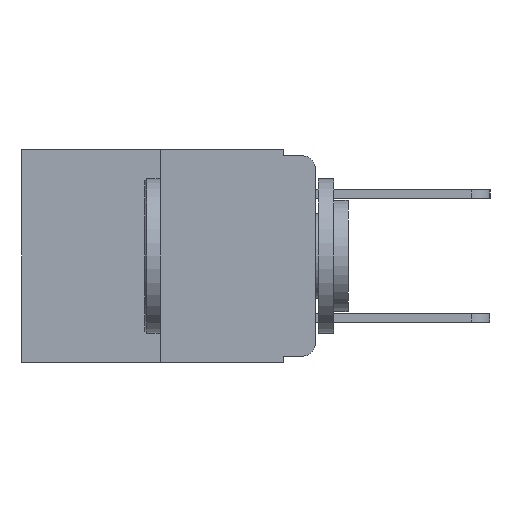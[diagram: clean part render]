
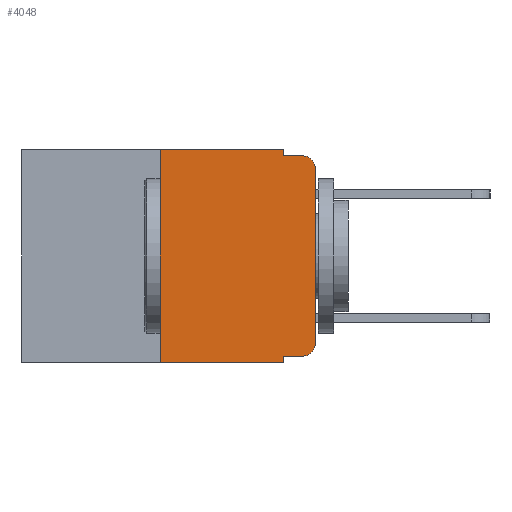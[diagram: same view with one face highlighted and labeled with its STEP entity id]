
A CAD part, left-side view. The second image highlights one B-rep face of the part: STEP entity #4048.
In plain terms, the highlighted planar face has unit normal (-1, 0, 0).
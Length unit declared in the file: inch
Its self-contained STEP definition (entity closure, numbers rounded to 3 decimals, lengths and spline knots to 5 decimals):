
#87 = DIRECTION ( 'NONE',  ( -1., 0., 0. ) ) ;
#447 = EDGE_CURVE ( 'NONE', #23786, #11235, #17488, .T. ) ;
#547 = ORIENTED_EDGE ( 'NONE', *, *, #9632, .F. ) ;
#900 = CARTESIAN_POINT ( 'NONE',  ( 0., 0.02, -0.01 ) ) ;
#1013 = EDGE_CURVE ( 'NONE', #1791, #23786, #21207, .T. ) ;
#1163 = CARTESIAN_POINT ( 'NONE',  ( 0., 0.473, 0. ) ) ;
#1171 = ORIENTED_EDGE ( 'NONE', *, *, #13634, .T. ) ;
#1400 = EDGE_CURVE ( 'NONE', #11235, #16687, #11119, .T. ) ;
#1454 = ORIENTED_EDGE ( 'NONE', *, *, #5997, .F. ) ;
#1662 = CARTESIAN_POINT ( 'NONE',  ( 0., 0.473, 0. ) ) ;
#1791 = VERTEX_POINT ( 'NONE', #5552 ) ;
#1856 = DIRECTION ( 'NONE',  ( 0., 0., -1. ) ) ;
#2005 = CARTESIAN_POINT ( 'NONE',  ( 0., 0.25, -0.343 ) ) ;
#2042 = DIRECTION ( 'NONE',  ( 0., 0., 1. ) ) ;
#2281 = AXIS2_PLACEMENT_3D ( 'NONE', #1163, #19923, #8902 ) ;
#2960 = CARTESIAN_POINT ( 'NONE',  ( 0., 0.051, -0.01 ) ) ;
#3100 = CARTESIAN_POINT ( 'NONE',  ( 0., 0., -0.313 ) ) ;
#3268 = ORIENTED_EDGE ( 'NONE', *, *, #447, .T. ) ;
#3965 = VERTEX_POINT ( 'NONE', #21559 ) ;
#4048 = ADVANCED_FACE ( 'NONE', ( #5320 ), #18096, .F. ) ;
#4071 = VECTOR ( 'NONE', #14919, 39.37008 ) ;
#4297 = CARTESIAN_POINT ( 'NONE',  ( 0., 0., -0.03 ) ) ;
#4522 = CARTESIAN_POINT ( 'NONE',  ( 0., 0., 0. ) ) ;
#4771 = EDGE_CURVE ( 'NONE', #18397, #10163, #5593, .T. ) ;
#5320 = FACE_OUTER_BOUND ( 'NONE', #21579, .T. ) ;
#5395 = CARTESIAN_POINT ( 'NONE',  ( 0., 0.02, -0.03 ) ) ;
#5552 = CARTESIAN_POINT ( 'NONE',  ( 0., 0.02, -0.333 ) ) ;
#5593 = LINE ( 'NONE', #11094, #17867 ) ;
#5877 = EDGE_CURVE ( 'NONE', #5978, #1791, #11521, .T. ) ;
#5978 = VERTEX_POINT ( 'NONE', #7218 ) ;
#5997 = EDGE_CURVE ( 'NONE', #10163, #3965, #8563, .T. ) ;
#6776 = CARTESIAN_POINT ( 'NONE',  ( 0., 0.051, -0.01 ) ) ;
#7046 = CARTESIAN_POINT ( 'NONE',  ( 0., 0.051, -0.333 ) ) ;
#7218 = CARTESIAN_POINT ( 'NONE',  ( 0., 0.051, -0.333 ) ) ;
#7567 = LINE ( 'NONE', #11397, #21168 ) ;
#7594 = DIRECTION ( 'NONE',  ( 0., 0., -1. ) ) ;
#7638 = EDGE_CURVE ( 'NONE', #3965, #18108, #23432, .T. ) ;
#8334 = EDGE_CURVE ( 'NONE', #5978, #15099, #7567, .T. ) ;
#8563 = LINE ( 'NONE', #1662, #4071 ) ;
#8730 = DIRECTION ( 'NONE',  ( 0., -1., 0. ) ) ;
#8902 = DIRECTION ( 'NONE',  ( 0., 0., -1. ) ) ;
#9164 = AXIS2_PLACEMENT_3D ( 'NONE', #5395, #20125, #12727 ) ;
#9280 = ORIENTED_EDGE ( 'NONE', *, *, #7638, .F. ) ;
#9632 = EDGE_CURVE ( 'NONE', #18108, #16687, #19071, .T. ) ;
#10147 = ORIENTED_EDGE ( 'NONE', *, *, #5877, .T. ) ;
#10163 = VERTEX_POINT ( 'NONE', #22997 ) ;
#10605 = CARTESIAN_POINT ( 'NONE',  ( 0., 0.473, -0.343 ) ) ;
#11094 = CARTESIAN_POINT ( 'NONE',  ( 0., 0.25, 0. ) ) ;
#11103 = CARTESIAN_POINT ( 'NONE',  ( 0., 0.051, -0.343 ) ) ;
#11119 = CIRCLE ( 'NONE', #9164, 0.02 ) ;
#11235 = VERTEX_POINT ( 'NONE', #4297 ) ;
#11349 = CARTESIAN_POINT ( 'NONE',  ( 0., 0.02, -0.313 ) ) ;
#11397 = CARTESIAN_POINT ( 'NONE',  ( 0., 0.051, 0. ) ) ;
#11521 = LINE ( 'NONE', #7046, #16972 ) ;
#12626 = VECTOR ( 'NONE', #2042, 39.37008 ) ;
#12727 = DIRECTION ( 'NONE',  ( 0., 0., -1. ) ) ;
#13193 = DIRECTION ( 'NONE',  ( 0., 0., -1. ) ) ;
#13634 = EDGE_CURVE ( 'NONE', #18397, #15099, #16624, .T. ) ;
#13745 = VECTOR ( 'NONE', #17985, 39.37008 ) ;
#13939 = ORIENTED_EDGE ( 'NONE', *, *, #4771, .F. ) ;
#14225 = VECTOR ( 'NONE', #8730, 39.37008 ) ;
#14798 = DIRECTION ( 'NONE',  ( 0., 0., 1. ) ) ;
#14919 = DIRECTION ( 'NONE',  ( 0., -1., 0. ) ) ;
#15099 = VERTEX_POINT ( 'NONE', #11103 ) ;
#16624 = LINE ( 'NONE', #10605, #13745 ) ;
#16687 = VERTEX_POINT ( 'NONE', #900 ) ;
#16972 = VECTOR ( 'NONE', #18170, 39.37008 ) ;
#17488 = LINE ( 'NONE', #4522, #12626 ) ;
#17867 = VECTOR ( 'NONE', #14798, 39.37008 ) ;
#17985 = DIRECTION ( 'NONE',  ( 0., -1., 0. ) ) ;
#18096 = PLANE ( 'NONE',  #2281 ) ;
#18108 = VERTEX_POINT ( 'NONE', #2960 ) ;
#18170 = DIRECTION ( 'NONE',  ( 0., -1., 0. ) ) ;
#18397 = VERTEX_POINT ( 'NONE', #2005 ) ;
#18585 = VECTOR ( 'NONE', #13193, 39.37008 ) ;
#19071 = LINE ( 'NONE', #6776, #14225 ) ;
#19923 = DIRECTION ( 'NONE',  ( 1., 0., 0. ) ) ;
#20125 = DIRECTION ( 'NONE',  ( -1., 0., 0. ) ) ;
#20495 = ORIENTED_EDGE ( 'NONE', *, *, #1013, .T. ) ;
#21168 = VECTOR ( 'NONE', #7594, 39.37008 ) ;
#21207 = CIRCLE ( 'NONE', #23588, 0.02 ) ;
#21559 = CARTESIAN_POINT ( 'NONE',  ( 0., 0.051, 0. ) ) ;
#21579 = EDGE_LOOP ( 'NONE', ( #3268, #23035, #547, #9280, #1454, #13939, #1171, #21684, #10147, #20495 ) ) ;
#21684 = ORIENTED_EDGE ( 'NONE', *, *, #8334, .F. ) ;
#22997 = CARTESIAN_POINT ( 'NONE',  ( 0., 0.25, 0. ) ) ;
#23035 = ORIENTED_EDGE ( 'NONE', *, *, #1400, .T. ) ;
#23432 = LINE ( 'NONE', #24119, #18585 ) ;
#23588 = AXIS2_PLACEMENT_3D ( 'NONE', #11349, #87, #1856 ) ;
#23786 = VERTEX_POINT ( 'NONE', #3100 ) ;
#24119 = CARTESIAN_POINT ( 'NONE',  ( 0., 0.051, 0. ) ) ;
